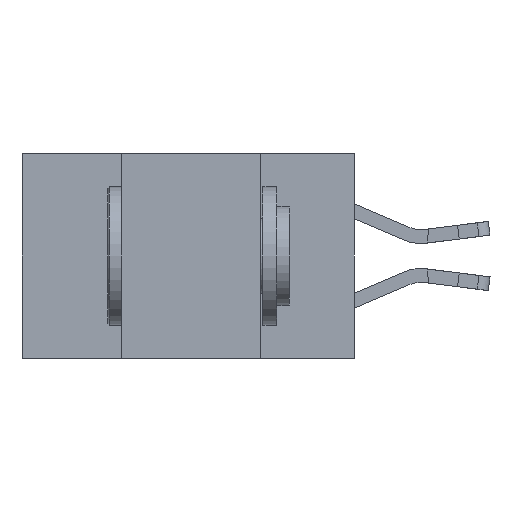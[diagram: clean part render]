
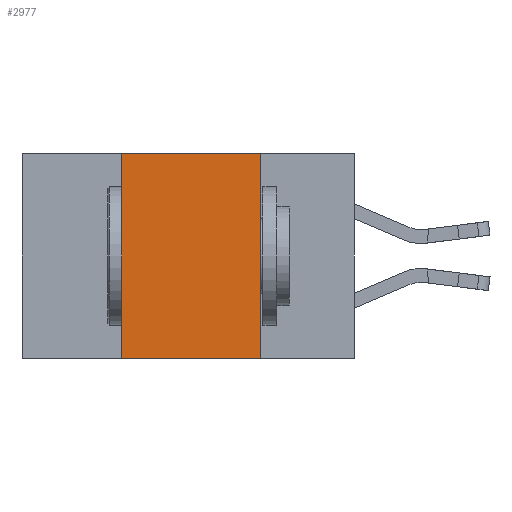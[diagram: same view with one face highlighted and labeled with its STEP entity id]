
A CAD part, left-side view. The second image highlights one B-rep face of the part: STEP entity #2977.
In plain terms, the highlighted planar face has unit normal (-1, 0, 0).
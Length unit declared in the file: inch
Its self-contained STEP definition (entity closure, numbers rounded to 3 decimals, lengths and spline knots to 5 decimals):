
#21 = CARTESIAN_POINT ( 'NONE',  ( 0., 0.17, -0.37 ) ) ;
#142 = AXIS2_PLACEMENT_3D ( 'NONE', #9111, #8505, #8488 ) ;
#834 = LINE ( 'NONE', #5812, #11805 ) ;
#1616 = VERTEX_POINT ( 'NONE', #12211 ) ;
#1793 = EDGE_CURVE ( 'NONE', #1616, #4940, #5006, .T. ) ;
#2004 = VERTEX_POINT ( 'NONE', #11492 ) ;
#2508 = EDGE_LOOP ( 'NONE', ( #12784, #4141, #7606, #3825 ) ) ;
#2737 = EDGE_CURVE ( 'NONE', #1616, #2004, #6357, .T. ) ;
#2977 = ADVANCED_FACE ( 'NONE', ( #18151 ), #8703, .F. ) ;
#3742 = EDGE_CURVE ( 'NONE', #2004, #15056, #8537, .T. ) ;
#3825 = ORIENTED_EDGE ( 'NONE', *, *, #1793, .T. ) ;
#3838 = CARTESIAN_POINT ( 'NONE',  ( 0., 0.6, 0. ) ) ;
#4115 = VECTOR ( 'NONE', #18232, 39.37008 ) ;
#4141 = ORIENTED_EDGE ( 'NONE', *, *, #3742, .F. ) ;
#4694 = EDGE_CURVE ( 'NONE', #15056, #4940, #834, .T. ) ;
#4940 = VERTEX_POINT ( 'NONE', #21 ) ;
#5006 = LINE ( 'NONE', #13118, #4115 ) ;
#5812 = CARTESIAN_POINT ( 'NONE',  ( 0., 0.17, -0.37 ) ) ;
#6357 = LINE ( 'NONE', #15687, #10126 ) ;
#7606 = ORIENTED_EDGE ( 'NONE', *, *, #2737, .F. ) ;
#8488 = DIRECTION ( 'NONE',  ( 0., 0., -1. ) ) ;
#8505 = DIRECTION ( 'NONE',  ( 1., 0., 0. ) ) ;
#8537 = LINE ( 'NONE', #3838, #15064 ) ;
#8703 = PLANE ( 'NONE',  #142 ) ;
#8816 = DIRECTION ( 'NONE',  ( 0., -1., 0. ) ) ;
#9111 = CARTESIAN_POINT ( 'NONE',  ( 0., 0.6, 0. ) ) ;
#10126 = VECTOR ( 'NONE', #15551, 39.37008 ) ;
#11492 = CARTESIAN_POINT ( 'NONE',  ( 0., 0.42, 0. ) ) ;
#11805 = VECTOR ( 'NONE', #16908, 39.37008 ) ;
#12211 = CARTESIAN_POINT ( 'NONE',  ( 0., 0.42, -0.37 ) ) ;
#12784 = ORIENTED_EDGE ( 'NONE', *, *, #4694, .F. ) ;
#13118 = CARTESIAN_POINT ( 'NONE',  ( 0., 0.6, -0.37 ) ) ;
#15056 = VERTEX_POINT ( 'NONE', #15582 ) ;
#15064 = VECTOR ( 'NONE', #8816, 39.37008 ) ;
#15551 = DIRECTION ( 'NONE',  ( 0., 0., 1. ) ) ;
#15582 = CARTESIAN_POINT ( 'NONE',  ( 0., 0.17, 0. ) ) ;
#15687 = CARTESIAN_POINT ( 'NONE',  ( 0., 0.42, -0.37 ) ) ;
#16908 = DIRECTION ( 'NONE',  ( 0., 0., -1. ) ) ;
#18151 = FACE_OUTER_BOUND ( 'NONE', #2508, .T. ) ;
#18232 = DIRECTION ( 'NONE',  ( 0., -1., 0. ) ) ;
